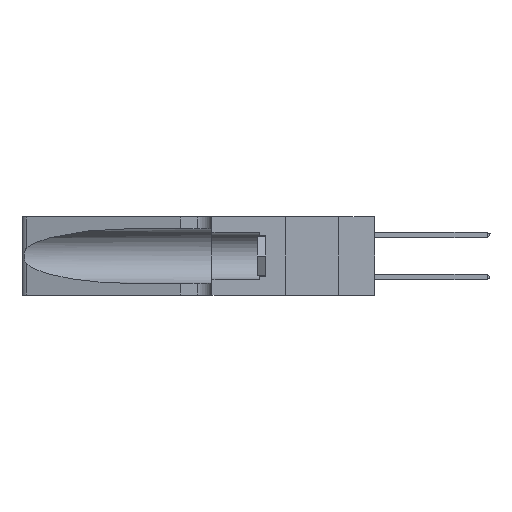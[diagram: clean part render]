
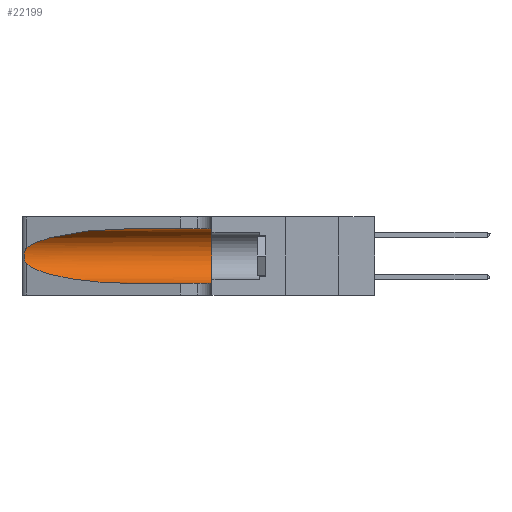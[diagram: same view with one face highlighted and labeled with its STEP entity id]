
A CAD part, left-side view. The second image highlights one B-rep face of the part: STEP entity #22199.
In plain terms, the highlighted cylindrical face has radius 3.308 mm (diameter 6.617 mm), a partial arc.
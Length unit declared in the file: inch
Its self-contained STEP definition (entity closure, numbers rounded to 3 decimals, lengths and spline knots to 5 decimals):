
#813 = CARTESIAN_POINT ( 'NONE',  ( 0.1305, 1.61858, 0.05475 ) ) ;
#973 = VERTEX_POINT ( 'NONE', #8400 ) ;
#1809 = CARTESIAN_POINT ( 'NONE',  ( 0.1305, 0.72297, 0.31525 ) ) ;
#1982 = CARTESIAN_POINT ( 'NONE',  ( 0.1305, 0.72297, 0.05475 ) ) ;
#2044 = EDGE_CURVE ( 'NONE', #2535, #11828, #11970, .T. ) ;
#2094 = CARTESIAN_POINT ( 'NONE',  ( 0.25555, 1.22993, 0.14849 ) ) ;
#2427 = EDGE_CURVE ( 'NONE', #11787, #2537, #14083, .T. ) ;
#2535 = VERTEX_POINT ( 'NONE', #1809 ) ;
#2537 = VERTEX_POINT ( 'NONE', #1982 ) ;
#3740 = EDGE_CURVE ( 'NONE', #2537, #973, #18620, .T. ) ;
#4074 = CARTESIAN_POINT ( 'NONE',  ( 0.25555, 1.22994, 0.2215 ) ) ;
#5859 = CARTESIAN_POINT ( 'NONE',  ( 0.1305, 0.72297, 0.05475 ) ) ;
#6171 = CARTESIAN_POINT ( 'NONE',  ( 0.25787, 1.23484, 0.2124 ) ) ;
#6380 = ORIENTED_EDGE ( 'NONE', *, *, #2427, .T. ) ;
#6685 = DIRECTION ( 'NONE',  ( 0., -1., 0. ) ) ;
#6768 = EDGE_LOOP ( 'NONE', ( #8193, #24023, #6380, #11886, #11900, #21662 ) ) ;
#6816 = CARTESIAN_POINT ( 'NONE',  ( 0.25487, 1.22718, 0.14631 ) ) ;
#7408 = CYLINDRICAL_SURFACE ( 'NONE', #10250, 0.13025 ) ;
#8193 = ORIENTED_EDGE ( 'NONE', *, *, #21891, .T. ) ;
#8253 = CARTESIAN_POINT ( 'NONE',  ( 0.26018, 1.23835, 0.19895 ) ) ;
#8400 = CARTESIAN_POINT ( 'NONE',  ( 0.1305, 0.35, 0.05475 ) ) ;
#9195 = CARTESIAN_POINT ( 'NONE',  ( 0.2373, 1.15595, 0.08982 ) ) ;
#9290 = B_SPLINE_CURVE_WITH_KNOTS ( 'NONE', 3,
 ( #14379, #4074, #18508, #6171, #20595, #8253, #22680, #10333, #24769, #12397, #16451, #14471, #2094, #16541 ),
 .UNSPECIFIED., .F., .F.,
 ( 4, 2, 2, 2, 2, 2, 4 ),
 ( 0., 0.00027, 0.00053, 0.00107, 0.0016, 0.00187, 0.00214 ),
 .UNSPECIFIED. ) ;
#9626 = EDGE_CURVE ( 'NONE', #22183, #11787, #9290, .T. ) ;
#9656 = CARTESIAN_POINT ( 'NONE',  ( 0.25487, 1.22718, 0.14631 ) ) ;
#9773 = CARTESIAN_POINT ( 'NONE',  ( 0.2373, 1.15595, 0.28018 ) ) ;
#9805 = EDGE_CURVE ( 'NONE', #11828, #973, #14002, .T. ) ;
#10250 = AXIS2_PLACEMENT_3D ( 'NONE', #23098, #10736, #25193 ) ;
#10333 = CARTESIAN_POINT ( 'NONE',  ( 0.26075, 1.23896, 0.178 ) ) ;
#10736 = DIRECTION ( 'NONE',  ( 0., -1., 0. ) ) ;
#10946 = CARTESIAN_POINT ( 'NONE',  ( 0.1305, 0.35, 0.185 ) ) ;
#11306 = VECTOR ( 'NONE', #6685, 39.37008 ) ;
#11787 = VERTEX_POINT ( 'NONE', #6816 ) ;
#11828 = VERTEX_POINT ( 'NONE', #19315 ) ;
#11886 = ORIENTED_EDGE ( 'NONE', *, *, #3740, .T. ) ;
#11900 = ORIENTED_EDGE ( 'NONE', *, *, #9805, .F. ) ;
#11970 = LINE ( 'NONE', #22421, #11306 ) ;
#12397 = CARTESIAN_POINT ( 'NONE',  ( 0.25856, 1.23593, 0.16098 ) ) ;
#13016 = DIRECTION ( 'NONE',  ( 0., 0., 1. ) ) ;
#13153 = VECTOR ( 'NONE', #17347, 39.37008 ) ;
#14002 = CIRCLE ( 'NONE', #17567, 0.13025 ) ;
#14083 =( BOUNDED_CURVE ( )  B_SPLINE_CURVE ( 3, ( #9656, #9195, #18024, #5859 ),
 .UNSPECIFIED., .F., .T. ) 
 B_SPLINE_CURVE_WITH_KNOTS ( ( 4, 4 ),
 ( 3.44316, 4.71239 ),
 .UNSPECIFIED. ) 
 CURVE ( )  GEOMETRIC_REPRESENTATION_ITEM ( )  RATIONAL_B_SPLINE_CURVE ( ( 1., 0.87, 0.87, 1. ) ) 
 REPRESENTATION_ITEM ( '' )  );
#14169 = FACE_OUTER_BOUND ( 'NONE', #6768, .T. ) ;
#14379 = CARTESIAN_POINT ( 'NONE',  ( 0.25487, 1.22718, 0.22369 ) ) ;
#14471 = CARTESIAN_POINT ( 'NONE',  ( 0.25639, 1.23186, 0.15144 ) ) ;
#16451 = CARTESIAN_POINT ( 'NONE',  ( 0.25789, 1.23486, 0.15765 ) ) ;
#16541 = CARTESIAN_POINT ( 'NONE',  ( 0.25487, 1.22718, 0.14631 ) ) ;
#17347 = DIRECTION ( 'NONE',  ( 0., -1., 0. ) ) ;
#17567 = AXIS2_PLACEMENT_3D ( 'NONE', #10946, #25397, #13016 ) ;
#17953 = CARTESIAN_POINT ( 'NONE',  ( 0.1305, 0.72297, 0.31525 ) ) ;
#18024 = CARTESIAN_POINT ( 'NONE',  ( 0.18966, 0.96281, 0.05475 ) ) ;
#18508 = CARTESIAN_POINT ( 'NONE',  ( 0.25639, 1.23184, 0.21858 ) ) ;
#18620 = LINE ( 'NONE', #813, #13153 ) ;
#18830 = CARTESIAN_POINT ( 'NONE',  ( 0.25487, 1.22718, 0.22369 ) ) ;
#19315 = CARTESIAN_POINT ( 'NONE',  ( 0.1305, 0.35, 0.31525 ) ) ;
#19687 =( BOUNDED_CURVE ( )  B_SPLINE_CURVE ( 3, ( #17953, #24110, #9773, #24205 ),
 .UNSPECIFIED., .F., .F. ) 
 B_SPLINE_CURVE_WITH_KNOTS ( ( 4, 4 ),
 ( 1.5708, 2.84003 ),
 .UNSPECIFIED. ) 
 CURVE ( )  GEOMETRIC_REPRESENTATION_ITEM ( )  RATIONAL_B_SPLINE_CURVE ( ( 1., 0.87, 0.87, 1. ) ) 
 REPRESENTATION_ITEM ( '' )  );
#20595 = CARTESIAN_POINT ( 'NONE',  ( 0.25854, 1.2359, 0.20912 ) ) ;
#21662 = ORIENTED_EDGE ( 'NONE', *, *, #2044, .F. ) ;
#21891 = EDGE_CURVE ( 'NONE', #2535, #22183, #19687, .T. ) ;
#22183 = VERTEX_POINT ( 'NONE', #18830 ) ;
#22199 = ADVANCED_FACE ( 'NONE', ( #14169 ), #7408, .F. ) ;
#22421 = CARTESIAN_POINT ( 'NONE',  ( 0.1305, 1.61858, 0.31525 ) ) ;
#22680 = CARTESIAN_POINT ( 'NONE',  ( 0.26075, 1.23896, 0.19203 ) ) ;
#23098 = CARTESIAN_POINT ( 'NONE',  ( 0.1305, 1.61858, 0.185 ) ) ;
#24023 = ORIENTED_EDGE ( 'NONE', *, *, #9626, .T. ) ;
#24110 = CARTESIAN_POINT ( 'NONE',  ( 0.18966, 0.96281, 0.31525 ) ) ;
#24205 = CARTESIAN_POINT ( 'NONE',  ( 0.25487, 1.22718, 0.22369 ) ) ;
#24769 = CARTESIAN_POINT ( 'NONE',  ( 0.26017, 1.23833, 0.17102 ) ) ;
#25193 = DIRECTION ( 'NONE',  ( 0., 0., -1. ) ) ;
#25397 = DIRECTION ( 'NONE',  ( 0., 1., 0. ) ) ;
